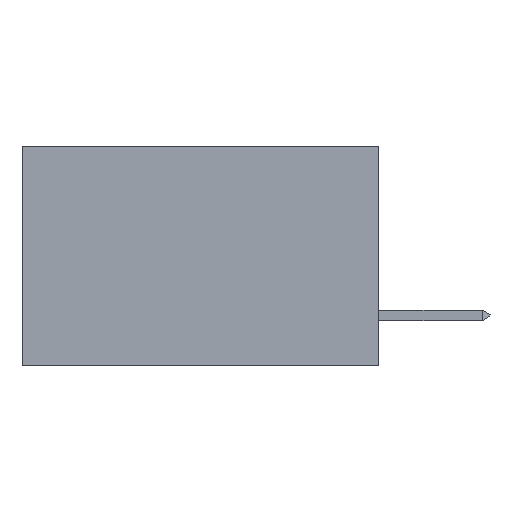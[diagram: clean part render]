
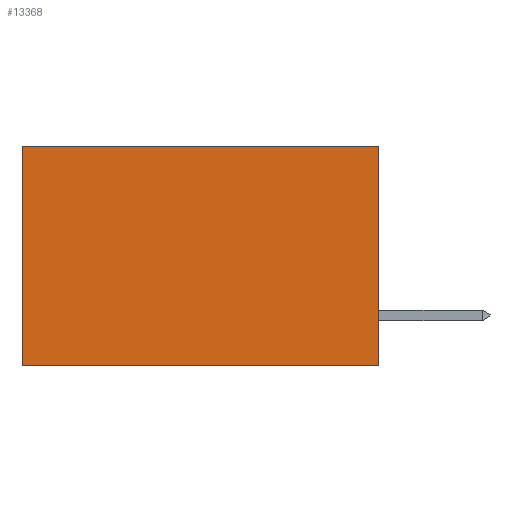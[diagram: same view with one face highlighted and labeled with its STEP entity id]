
A CAD part, left-side view. The second image highlights one B-rep face of the part: STEP entity #13368.
In plain terms, the highlighted planar face has unit normal (-1, 0, 0).
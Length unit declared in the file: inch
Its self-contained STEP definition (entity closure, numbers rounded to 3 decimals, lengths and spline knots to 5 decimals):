
#597 = ORIENTED_EDGE ( 'NONE', *, *, #12446, .F. ) ;
#1278 = CARTESIAN_POINT ( 'NONE',  ( 0.2615, 0., 0. ) ) ;
#1714 = DIRECTION ( 'NONE',  ( 1., 0., 0. ) ) ;
#1753 = DIRECTION ( 'NONE',  ( 0., 1., 0. ) ) ;
#2008 = LINE ( 'NONE', #4930, #13108 ) ;
#2119 = EDGE_CURVE ( 'NONE', #4059, #10592, #7638, .T. ) ;
#2787 = CARTESIAN_POINT ( 'NONE',  ( 0.2615, 0., -0.37 ) ) ;
#3186 = CARTESIAN_POINT ( 'NONE',  ( 0.2615, 0.6, 0. ) ) ;
#3526 = CARTESIAN_POINT ( 'NONE',  ( 0.2615, 0.6, -0.37 ) ) ;
#3629 = CARTESIAN_POINT ( 'NONE',  ( 0.2615, 0., -0.37 ) ) ;
#3738 = AXIS2_PLACEMENT_3D ( 'NONE', #11522, #1714, #8080 ) ;
#4059 = VERTEX_POINT ( 'NONE', #3186 ) ;
#4569 = EDGE_CURVE ( 'NONE', #4855, #10592, #7077, .T. ) ;
#4600 = CARTESIAN_POINT ( 'NONE',  ( 0.2615, 0., -0.37 ) ) ;
#4855 = VERTEX_POINT ( 'NONE', #3629 ) ;
#4930 = CARTESIAN_POINT ( 'NONE',  ( 0.2615, 0., 0. ) ) ;
#5478 = VECTOR ( 'NONE', #8519, 39.37008 ) ;
#5649 = DIRECTION ( 'NONE',  ( 0., 0., -1. ) ) ;
#6590 = EDGE_LOOP ( 'NONE', ( #6883, #12845, #597, #10509 ) ) ;
#6655 = EDGE_CURVE ( 'NONE', #7016, #4059, #2008, .T. ) ;
#6883 = ORIENTED_EDGE ( 'NONE', *, *, #2119, .T. ) ;
#7016 = VERTEX_POINT ( 'NONE', #1278 ) ;
#7042 = DIRECTION ( 'NONE',  ( 0., 1., 0. ) ) ;
#7077 = LINE ( 'NONE', #2787, #13694 ) ;
#7523 = CARTESIAN_POINT ( 'NONE',  ( 0.2615, 0.6, -0.37 ) ) ;
#7638 = LINE ( 'NONE', #7523, #5478 ) ;
#8080 = DIRECTION ( 'NONE',  ( 0., 0., -1. ) ) ;
#8519 = DIRECTION ( 'NONE',  ( 0., 0., -1. ) ) ;
#8534 = VECTOR ( 'NONE', #5649, 39.37008 ) ;
#9258 = PLANE ( 'NONE',  #3738 ) ;
#9857 = FACE_OUTER_BOUND ( 'NONE', #6590, .T. ) ;
#10509 = ORIENTED_EDGE ( 'NONE', *, *, #6655, .T. ) ;
#10561 = LINE ( 'NONE', #4600, #8534 ) ;
#10592 = VERTEX_POINT ( 'NONE', #3526 ) ;
#11522 = CARTESIAN_POINT ( 'NONE',  ( 0.2615, 0., -0.37 ) ) ;
#12446 = EDGE_CURVE ( 'NONE', #7016, #4855, #10561, .T. ) ;
#12845 = ORIENTED_EDGE ( 'NONE', *, *, #4569, .F. ) ;
#13108 = VECTOR ( 'NONE', #7042, 39.37008 ) ;
#13368 = ADVANCED_FACE ( 'NONE', ( #9857 ), #9258, .F. ) ;
#13694 = VECTOR ( 'NONE', #1753, 39.37008 ) ;
